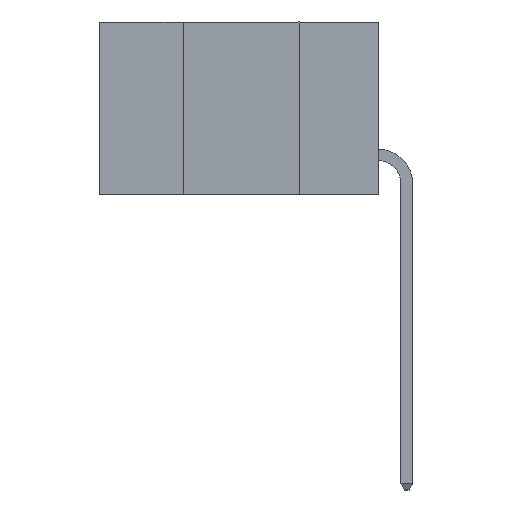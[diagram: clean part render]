
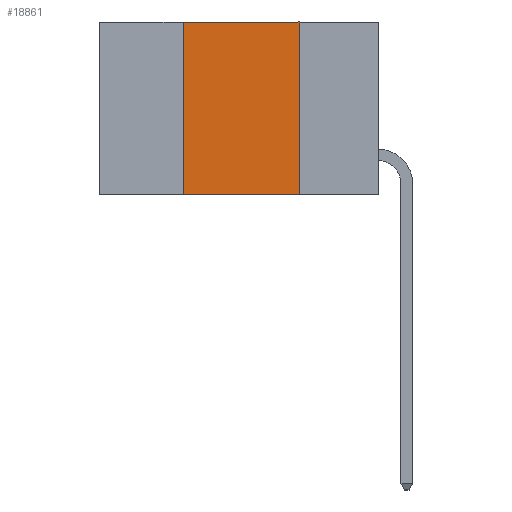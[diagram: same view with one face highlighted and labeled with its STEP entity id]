
A CAD part, left-side view. The second image highlights one B-rep face of the part: STEP entity #18861.
In plain terms, the highlighted planar face has unit normal (-1, 0, 0).
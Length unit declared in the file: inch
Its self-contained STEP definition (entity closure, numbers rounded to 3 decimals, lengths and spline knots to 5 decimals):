
#73 = VECTOR ( 'NONE', #19340, 39.37008 ) ;
#357 = VECTOR ( 'NONE', #15476, 39.37008 ) ;
#863 = LINE ( 'NONE', #15519, #357 ) ;
#3856 = ORIENTED_EDGE ( 'NONE', *, *, #10142, .F. ) ;
#5348 = LINE ( 'NONE', #11423, #9495 ) ;
#5446 = CARTESIAN_POINT ( 'NONE',  ( 0., 0.6, 0. ) ) ;
#5633 = VERTEX_POINT ( 'NONE', #6532 ) ;
#5722 = LINE ( 'NONE', #6068, #9374 ) ;
#6068 = CARTESIAN_POINT ( 'NONE',  ( 0., 0.17, -0.37 ) ) ;
#6150 = DIRECTION ( 'NONE',  ( 0., 0., -1. ) ) ;
#6311 = ORIENTED_EDGE ( 'NONE', *, *, #9096, .F. ) ;
#6322 = AXIS2_PLACEMENT_3D ( 'NONE', #5446, #16304, #7032 ) ;
#6532 = CARTESIAN_POINT ( 'NONE',  ( 0., 0.42, 0. ) ) ;
#6808 = ORIENTED_EDGE ( 'NONE', *, *, #18774, .F. ) ;
#7032 = DIRECTION ( 'NONE',  ( 0., 0., -1. ) ) ;
#7388 = CARTESIAN_POINT ( 'NONE',  ( 0., 0.42, -0.37 ) ) ;
#9096 = EDGE_CURVE ( 'NONE', #15518, #5633, #863, .T. ) ;
#9113 = VERTEX_POINT ( 'NONE', #15293 ) ;
#9308 = VERTEX_POINT ( 'NONE', #13543 ) ;
#9374 = VECTOR ( 'NONE', #6150, 39.37008 ) ;
#9495 = VECTOR ( 'NONE', #13004, 39.37008 ) ;
#10142 = EDGE_CURVE ( 'NONE', #9308, #9113, #5722, .T. ) ;
#11423 = CARTESIAN_POINT ( 'NONE',  ( 0., 0.6, 0. ) ) ;
#12021 = LINE ( 'NONE', #17795, #73 ) ;
#13004 = DIRECTION ( 'NONE',  ( 0., -1., 0. ) ) ;
#13197 = EDGE_CURVE ( 'NONE', #15518, #9113, #12021, .T. ) ;
#13543 = CARTESIAN_POINT ( 'NONE',  ( 0., 0.17, 0. ) ) ;
#15293 = CARTESIAN_POINT ( 'NONE',  ( 0., 0.17, -0.37 ) ) ;
#15476 = DIRECTION ( 'NONE',  ( 0., 0., 1. ) ) ;
#15518 = VERTEX_POINT ( 'NONE', #7388 ) ;
#15519 = CARTESIAN_POINT ( 'NONE',  ( 0., 0.42, -0.37 ) ) ;
#16304 = DIRECTION ( 'NONE',  ( 1., 0., 0. ) ) ;
#16514 = ORIENTED_EDGE ( 'NONE', *, *, #13197, .T. ) ;
#17795 = CARTESIAN_POINT ( 'NONE',  ( 0., 0.6, -0.37 ) ) ;
#18774 = EDGE_CURVE ( 'NONE', #5633, #9308, #5348, .T. ) ;
#18861 = ADVANCED_FACE ( 'NONE', ( #19398 ), #19334, .F. ) ;
#19334 = PLANE ( 'NONE',  #6322 ) ;
#19340 = DIRECTION ( 'NONE',  ( 0., -1., 0. ) ) ;
#19398 = FACE_OUTER_BOUND ( 'NONE', #19479, .T. ) ;
#19479 = EDGE_LOOP ( 'NONE', ( #3856, #6808, #6311, #16514 ) ) ;
